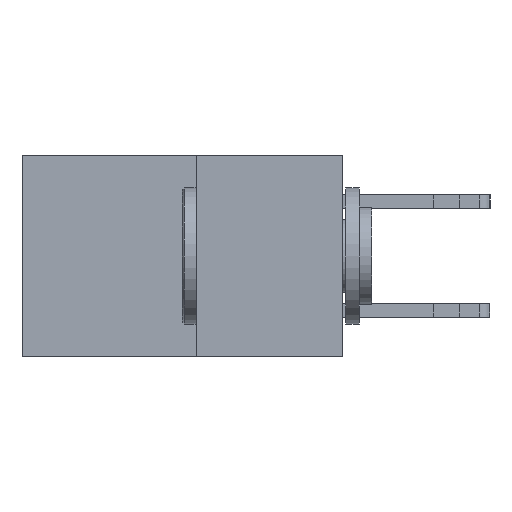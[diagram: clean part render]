
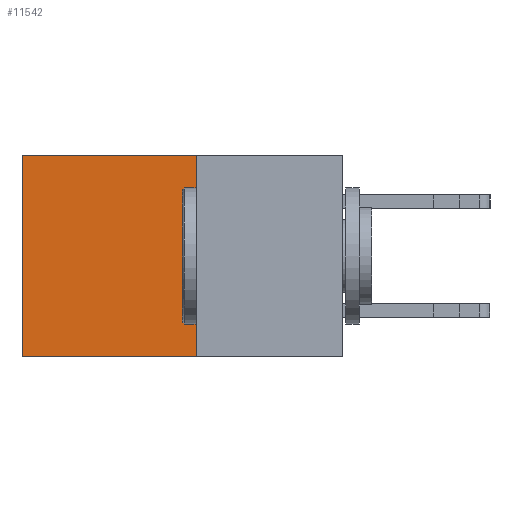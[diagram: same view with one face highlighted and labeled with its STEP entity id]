
A CAD part, left-side view. The second image highlights one B-rep face of the part: STEP entity #11542.
In plain terms, the highlighted planar face has unit normal (-1, 0, 0).
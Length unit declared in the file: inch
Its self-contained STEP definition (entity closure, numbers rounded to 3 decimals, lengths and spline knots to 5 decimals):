
#238 = DIRECTION ( 'NONE',  ( 0., 1., 0. ) ) ;
#397 = EDGE_CURVE ( 'NONE', #6417, #2370, #10958, .T. ) ;
#468 = AXIS2_PLACEMENT_3D ( 'NONE', #27591, #15792, #1600 ) ;
#1392 = EDGE_CURVE ( 'NONE', #29438, #2370, #7950, .T. ) ;
#1600 = DIRECTION ( 'NONE',  ( 0., 0., -1. ) ) ;
#1625 = VECTOR ( 'NONE', #238, 39.37008 ) ;
#2370 = VERTEX_POINT ( 'NONE', #7313 ) ;
#2484 = EDGE_LOOP ( 'NONE', ( #3299, #4491, #16616, #8776 ) ) ;
#2794 = FACE_OUTER_BOUND ( 'NONE', #2484, .T. ) ;
#3299 = ORIENTED_EDGE ( 'NONE', *, *, #397, .T. ) ;
#4491 = ORIENTED_EDGE ( 'NONE', *, *, #1392, .F. ) ;
#4666 = VECTOR ( 'NONE', #20310, 39.37008 ) ;
#6417 = VERTEX_POINT ( 'NONE', #26834 ) ;
#7313 = CARTESIAN_POINT ( 'NONE',  ( 0.277, 0.59, -0.37 ) ) ;
#7797 = LINE ( 'NONE', #15945, #25917 ) ;
#7892 = CARTESIAN_POINT ( 'NONE',  ( 0.277, 0.27, -0.37 ) ) ;
#7950 = LINE ( 'NONE', #7892, #1625 ) ;
#8776 = ORIENTED_EDGE ( 'NONE', *, *, #18269, .T. ) ;
#9046 = LINE ( 'NONE', #17018, #21716 ) ;
#10958 = LINE ( 'NONE', #15515, #4666 ) ;
#11542 = ADVANCED_FACE ( 'NONE', ( #2794 ), #29909, .F. ) ;
#15132 = EDGE_CURVE ( 'NONE', #20741, #29438, #7797, .T. ) ;
#15515 = CARTESIAN_POINT ( 'NONE',  ( 0.277, 0.59, -0.37 ) ) ;
#15792 = DIRECTION ( 'NONE',  ( 1., 0., 0. ) ) ;
#15945 = CARTESIAN_POINT ( 'NONE',  ( 0.277, 0.27, -0.37 ) ) ;
#16616 = ORIENTED_EDGE ( 'NONE', *, *, #15132, .F. ) ;
#17018 = CARTESIAN_POINT ( 'NONE',  ( 0.277, 0.27, 0. ) ) ;
#18269 = EDGE_CURVE ( 'NONE', #20741, #6417, #9046, .T. ) ;
#18376 = DIRECTION ( 'NONE',  ( 0., 0., -1. ) ) ;
#18512 = CARTESIAN_POINT ( 'NONE',  ( 0.277, 0.27, 0. ) ) ;
#19427 = DIRECTION ( 'NONE',  ( 0., 1., 0. ) ) ;
#20310 = DIRECTION ( 'NONE',  ( 0., 0., -1. ) ) ;
#20741 = VERTEX_POINT ( 'NONE', #18512 ) ;
#21716 = VECTOR ( 'NONE', #19427, 39.37008 ) ;
#25917 = VECTOR ( 'NONE', #18376, 39.37008 ) ;
#26834 = CARTESIAN_POINT ( 'NONE',  ( 0.277, 0.59, 0. ) ) ;
#27591 = CARTESIAN_POINT ( 'NONE',  ( 0.277, 0.27, -0.37 ) ) ;
#29438 = VERTEX_POINT ( 'NONE', #29558 ) ;
#29558 = CARTESIAN_POINT ( 'NONE',  ( 0.277, 0.27, -0.37 ) ) ;
#29909 = PLANE ( 'NONE',  #468 ) ;
